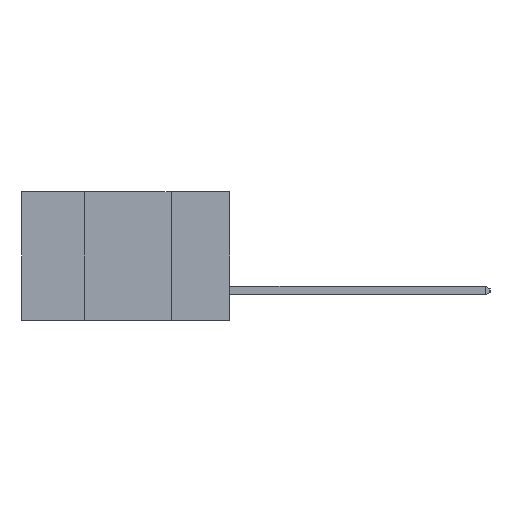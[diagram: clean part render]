
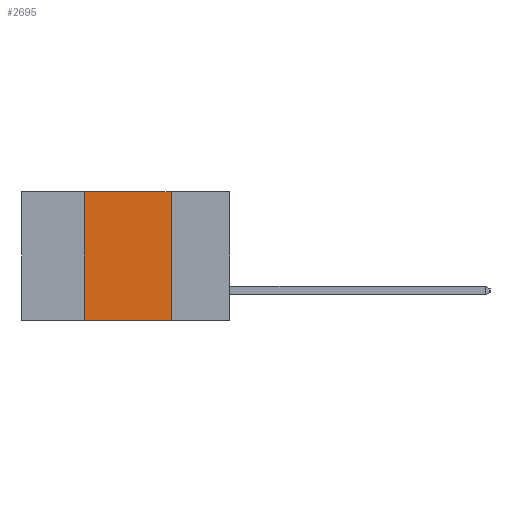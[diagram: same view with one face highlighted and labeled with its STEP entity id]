
A CAD part, left-side view. The second image highlights one B-rep face of the part: STEP entity #2695.
In plain terms, the highlighted planar face has unit normal (-1, 0, 0).
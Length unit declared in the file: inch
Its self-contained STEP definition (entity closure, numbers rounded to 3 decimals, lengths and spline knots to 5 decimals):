
#232 = CARTESIAN_POINT ( 'NONE',  ( 0., 0.6, -0.37 ) ) ;
#347 = CARTESIAN_POINT ( 'NONE',  ( 0., 0.42, -0.37 ) ) ;
#458 = VERTEX_POINT ( 'NONE', #1593 ) ;
#1080 = ORIENTED_EDGE ( 'NONE', *, *, #7463, .F. ) ;
#1281 = CARTESIAN_POINT ( 'NONE',  ( 0., 0.17, 0. ) ) ;
#1330 = CARTESIAN_POINT ( 'NONE',  ( 0., 0.6, 0. ) ) ;
#1593 = CARTESIAN_POINT ( 'NONE',  ( 0., 0.17, -0.37 ) ) ;
#1841 = VERTEX_POINT ( 'NONE', #12291 ) ;
#1943 = LINE ( 'NONE', #1330, #11691 ) ;
#2149 = CARTESIAN_POINT ( 'NONE',  ( 0., 0.42, -0.37 ) ) ;
#2603 = DIRECTION ( 'NONE',  ( 0., -1., 0. ) ) ;
#2695 = ADVANCED_FACE ( 'NONE', ( #7875 ), #9221, .F. ) ;
#3210 = LINE ( 'NONE', #2149, #12628 ) ;
#5567 = DIRECTION ( 'NONE',  ( 1., 0., 0. ) ) ;
#5587 = EDGE_CURVE ( 'NONE', #11693, #458, #11311, .T. ) ;
#5940 = CARTESIAN_POINT ( 'NONE',  ( 0., 0.17, -0.37 ) ) ;
#6242 = EDGE_CURVE ( 'NONE', #11693, #1841, #3210, .T. ) ;
#6644 = ORIENTED_EDGE ( 'NONE', *, *, #6860, .F. ) ;
#6860 = EDGE_CURVE ( 'NONE', #1841, #10341, #1943, .T. ) ;
#6935 = AXIS2_PLACEMENT_3D ( 'NONE', #11000, #5567, #11861 ) ;
#6946 = ORIENTED_EDGE ( 'NONE', *, *, #5587, .T. ) ;
#7403 = EDGE_LOOP ( 'NONE', ( #1080, #6644, #11400, #6946 ) ) ;
#7463 = EDGE_CURVE ( 'NONE', #10341, #458, #10731, .T. ) ;
#7875 = FACE_OUTER_BOUND ( 'NONE', #7403, .T. ) ;
#8365 = VECTOR ( 'NONE', #9626, 39.37008 ) ;
#8474 = DIRECTION ( 'NONE',  ( 0., -1., 0. ) ) ;
#8958 = VECTOR ( 'NONE', #8474, 39.37008 ) ;
#9221 = PLANE ( 'NONE',  #6935 ) ;
#9626 = DIRECTION ( 'NONE',  ( 0., 0., -1. ) ) ;
#10341 = VERTEX_POINT ( 'NONE', #1281 ) ;
#10731 = LINE ( 'NONE', #5940, #8365 ) ;
#11000 = CARTESIAN_POINT ( 'NONE',  ( 0., 0.6, 0. ) ) ;
#11311 = LINE ( 'NONE', #232, #8958 ) ;
#11400 = ORIENTED_EDGE ( 'NONE', *, *, #6242, .F. ) ;
#11691 = VECTOR ( 'NONE', #2603, 39.37008 ) ;
#11693 = VERTEX_POINT ( 'NONE', #347 ) ;
#11861 = DIRECTION ( 'NONE',  ( 0., 0., -1. ) ) ;
#12291 = CARTESIAN_POINT ( 'NONE',  ( 0., 0.42, 0. ) ) ;
#12380 = DIRECTION ( 'NONE',  ( 0., 0., 1. ) ) ;
#12628 = VECTOR ( 'NONE', #12380, 39.37008 ) ;
